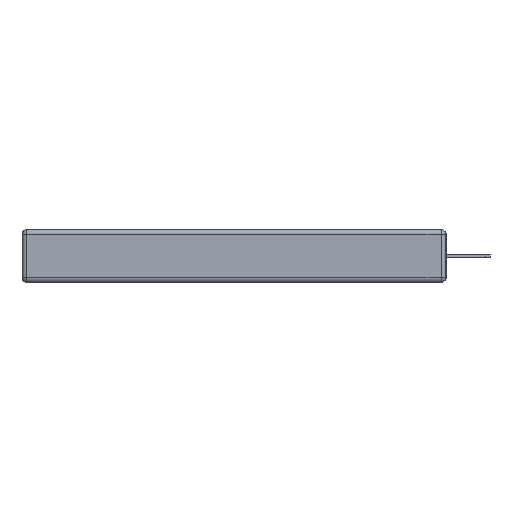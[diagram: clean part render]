
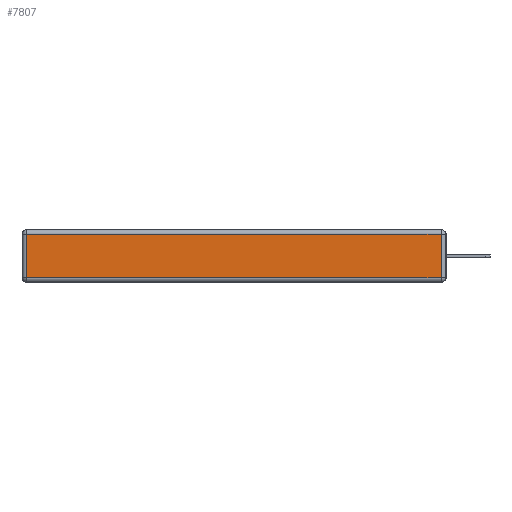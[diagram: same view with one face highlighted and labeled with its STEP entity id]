
A CAD part, left-side view. The second image highlights one B-rep face of the part: STEP entity #7807.
In plain terms, the highlighted planar face has unit normal (-1, 0, 0).
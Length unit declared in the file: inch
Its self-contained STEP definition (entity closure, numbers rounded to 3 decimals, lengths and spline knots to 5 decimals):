
#563 = DIRECTION ( 'NONE',  ( -1., 0., 0. ) ) ;
#672 = DIRECTION ( 'NONE',  ( 0., 0., 1. ) ) ;
#924 = VECTOR ( 'NONE', #13978, 39.37008 ) ;
#4174 = VECTOR ( 'NONE', #16424, 39.37008 ) ;
#4197 = DIRECTION ( 'NONE',  ( 0., 0., -1. ) ) ;
#4241 = DIRECTION ( 'NONE',  ( 0., -1., 0. ) ) ;
#4542 = LINE ( 'NONE', #19597, #19226 ) ;
#5147 = ORIENTED_EDGE ( 'NONE', *, *, #19073, .T. ) ;
#5855 = ORIENTED_EDGE ( 'NONE', *, *, #19558, .T. ) ;
#6431 = PLANE ( 'NONE',  #13929 ) ;
#6866 = VECTOR ( 'NONE', #4197, 39.37008 ) ;
#7194 = LINE ( 'NONE', #10366, #4174 ) ;
#7691 = CARTESIAN_POINT ( 'NONE',  ( 0., 2.72, -0.03 ) ) ;
#7770 = EDGE_CURVE ( 'NONE', #17300, #8666, #8115, .T. ) ;
#7807 = ADVANCED_FACE ( 'NONE', ( #14161 ), #6431, .T. ) ;
#8115 = LINE ( 'NONE', #11093, #924 ) ;
#8569 = CARTESIAN_POINT ( 'NONE',  ( 0., 0.03, -0.03 ) ) ;
#8666 = VERTEX_POINT ( 'NONE', #7691 ) ;
#9421 = ORIENTED_EDGE ( 'NONE', *, *, #16868, .T. ) ;
#9773 = VERTEX_POINT ( 'NONE', #14061 ) ;
#10366 = CARTESIAN_POINT ( 'NONE',  ( 0., 0.03, -0.343 ) ) ;
#11093 = CARTESIAN_POINT ( 'NONE',  ( 0., 2.75, -0.03 ) ) ;
#11505 = CARTESIAN_POINT ( 'NONE',  ( 0., 2.72, -0.343 ) ) ;
#11701 = LINE ( 'NONE', #11505, #6866 ) ;
#13918 = CARTESIAN_POINT ( 'NONE',  ( 0., 2.72, -0.313 ) ) ;
#13929 = AXIS2_PLACEMENT_3D ( 'NONE', #18527, #563, #672 ) ;
#13978 = DIRECTION ( 'NONE',  ( 0., 1., 0. ) ) ;
#14061 = CARTESIAN_POINT ( 'NONE',  ( 0., 0.03, -0.313 ) ) ;
#14161 = FACE_OUTER_BOUND ( 'NONE', #17746, .T. ) ;
#16424 = DIRECTION ( 'NONE',  ( 0., 0., 1. ) ) ;
#16868 = EDGE_CURVE ( 'NONE', #9773, #17300, #7194, .T. ) ;
#17077 = VERTEX_POINT ( 'NONE', #13918 ) ;
#17300 = VERTEX_POINT ( 'NONE', #8569 ) ;
#17746 = EDGE_LOOP ( 'NONE', ( #5855, #9421, #17836, #5147 ) ) ;
#17836 = ORIENTED_EDGE ( 'NONE', *, *, #7770, .T. ) ;
#18527 = CARTESIAN_POINT ( 'NONE',  ( 0., 0., -0.343 ) ) ;
#19073 = EDGE_CURVE ( 'NONE', #8666, #17077, #11701, .T. ) ;
#19226 = VECTOR ( 'NONE', #4241, 39.37008 ) ;
#19558 = EDGE_CURVE ( 'NONE', #17077, #9773, #4542, .T. ) ;
#19597 = CARTESIAN_POINT ( 'NONE',  ( 0., 0., -0.313 ) ) ;
